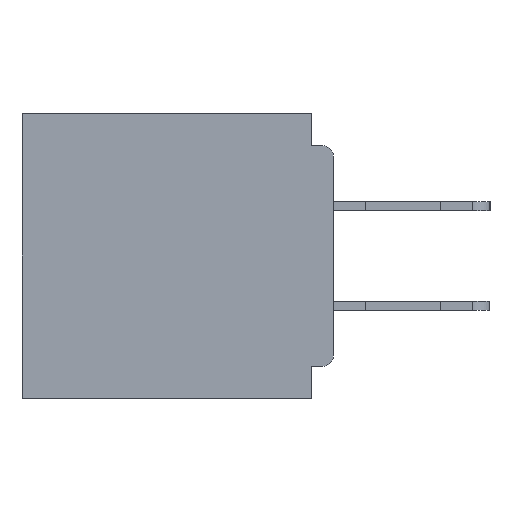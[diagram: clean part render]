
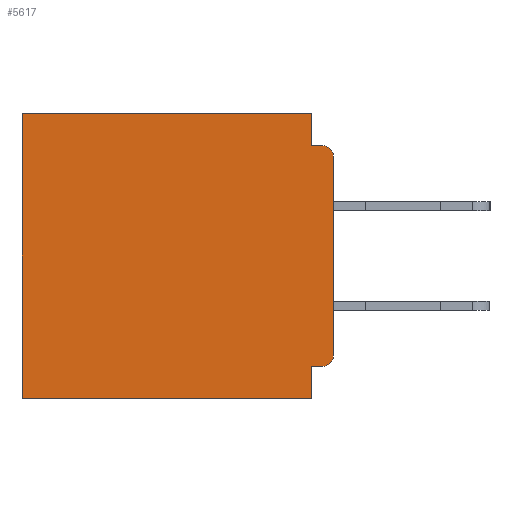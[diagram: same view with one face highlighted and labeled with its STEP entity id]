
A CAD part, left-side view. The second image highlights one B-rep face of the part: STEP entity #5617.
In plain terms, the highlighted planar face has unit normal (-1, 0, 0).
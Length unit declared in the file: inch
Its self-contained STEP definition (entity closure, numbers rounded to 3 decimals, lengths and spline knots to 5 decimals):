
#1037 = LINE ( 'NONE', #33477, #38557 ) ;
#1380 = DIRECTION ( 'NONE',  ( 0., -1., 0. ) ) ;
#1863 = EDGE_CURVE ( 'NONE', #27059, #33455, #26559, .T. ) ;
#2200 = DIRECTION ( 'NONE',  ( 1., 0., 0. ) ) ;
#4066 = EDGE_CURVE ( 'NONE', #7478, #38044, #1037, .T. ) ;
#4143 = CARTESIAN_POINT ( 'NONE',  ( 0.3, 0.015, -0.34 ) ) ;
#4720 = VERTEX_POINT ( 'NONE', #11070 ) ;
#5083 = FACE_OUTER_BOUND ( 'NONE', #17525, .T. ) ;
#5617 = ADVANCED_FACE ( 'NONE', ( #5083 ), #24714, .F. ) ;
#6187 = CARTESIAN_POINT ( 'NONE',  ( 0.3, 0., -0.4 ) ) ;
#6511 = CIRCLE ( 'NONE', #29868, 0.015 ) ;
#6643 = VERTEX_POINT ( 'NONE', #28253 ) ;
#7478 = VERTEX_POINT ( 'NONE', #33227 ) ;
#8003 = DIRECTION ( 'NONE',  ( 0., 0., -1. ) ) ;
#8514 = LINE ( 'NONE', #6187, #18417 ) ;
#8592 = EDGE_CURVE ( 'NONE', #28787, #31553, #8514, .T. ) ;
#9430 = CARTESIAN_POINT ( 'NONE',  ( 0.3, 0., -0.355 ) ) ;
#9519 = EDGE_CURVE ( 'NONE', #28787, #46571, #16006, .T. ) ;
#9896 = DIRECTION ( 'NONE',  ( 0., 1., 0. ) ) ;
#11070 = CARTESIAN_POINT ( 'NONE',  ( 0.3, 0.031, -0.355 ) ) ;
#11517 = ORIENTED_EDGE ( 'NONE', *, *, #4066, .F. ) ;
#15124 = CARTESIAN_POINT ( 'NONE',  ( 0.3, 0., -0.06 ) ) ;
#15495 = VECTOR ( 'NONE', #15635, 39.37008 ) ;
#15635 = DIRECTION ( 'NONE',  ( 0., 1., 0. ) ) ;
#16006 = CIRCLE ( 'NONE', #46215, 0.015 ) ;
#16523 = LINE ( 'NONE', #28769, #35234 ) ;
#17525 = EDGE_LOOP ( 'NONE', ( #47558, #17944, #19115, #11517, #26168, #48163, #24986, #31431, #34925, #23362 ) ) ;
#17944 = ORIENTED_EDGE ( 'NONE', *, *, #9519, .T. ) ;
#18105 = CARTESIAN_POINT ( 'NONE',  ( 0.3, 0.015, -0.06 ) ) ;
#18132 = LINE ( 'NONE', #9430, #26917 ) ;
#18162 = CARTESIAN_POINT ( 'NONE',  ( 0.3, 0., -0.34 ) ) ;
#18417 = VECTOR ( 'NONE', #32317, 39.37008 ) ;
#19115 = ORIENTED_EDGE ( 'NONE', *, *, #44430, .F. ) ;
#19328 = CARTESIAN_POINT ( 'NONE',  ( 0.3, 0.437, -0.4 ) ) ;
#19511 = EDGE_CURVE ( 'NONE', #30591, #4720, #18132, .T. ) ;
#20132 = VECTOR ( 'NONE', #9896, 39.37008 ) ;
#20237 = DIRECTION ( 'NONE',  ( 0., 0., -1. ) ) ;
#20951 = CARTESIAN_POINT ( 'NONE',  ( 0.3, 0., -0.4 ) ) ;
#21867 = DIRECTION ( 'NONE',  ( 0., 0., -1. ) ) ;
#22524 = CARTESIAN_POINT ( 'NONE',  ( 0.3, 0.031, -0.045 ) ) ;
#22567 = VECTOR ( 'NONE', #1380, 39.37008 ) ;
#23362 = ORIENTED_EDGE ( 'NONE', *, *, #47787, .T. ) ;
#23904 = CARTESIAN_POINT ( 'NONE',  ( 0.3, 0., -0.045 ) ) ;
#24247 = LINE ( 'NONE', #37978, #15495 ) ;
#24714 = PLANE ( 'NONE',  #38413 ) ;
#24986 = ORIENTED_EDGE ( 'NONE', *, *, #45618, .F. ) ;
#26168 = ORIENTED_EDGE ( 'NONE', *, *, #45929, .T. ) ;
#26559 = LINE ( 'NONE', #19328, #43955 ) ;
#26917 = VECTOR ( 'NONE', #39247, 39.37008 ) ;
#27059 = VERTEX_POINT ( 'NONE', #38459 ) ;
#28253 = CARTESIAN_POINT ( 'NONE',  ( 0.3, 0.031, -0.4 ) ) ;
#28473 = DIRECTION ( 'NONE',  ( 0., 0., -1. ) ) ;
#28769 = CARTESIAN_POINT ( 'NONE',  ( 0.3, 0.031, -0.4 ) ) ;
#28787 = VERTEX_POINT ( 'NONE', #15124 ) ;
#29868 = AXIS2_PLACEMENT_3D ( 'NONE', #4143, #30381, #8003 ) ;
#30093 = LINE ( 'NONE', #46945, #20132 ) ;
#30145 = EDGE_CURVE ( 'NONE', #4720, #6643, #16523, .T. ) ;
#30381 = DIRECTION ( 'NONE',  ( -1., 0., 0. ) ) ;
#30591 = VERTEX_POINT ( 'NONE', #38644 ) ;
#31431 = ORIENTED_EDGE ( 'NONE', *, *, #30145, .F. ) ;
#31553 = VERTEX_POINT ( 'NONE', #18162 ) ;
#32317 = DIRECTION ( 'NONE',  ( 0., 0., -1. ) ) ;
#32508 = DIRECTION ( 'NONE',  ( 0., 0., -1. ) ) ;
#33227 = CARTESIAN_POINT ( 'NONE',  ( 0.3, 0.031, 0. ) ) ;
#33455 = VERTEX_POINT ( 'NONE', #37112 ) ;
#33477 = CARTESIAN_POINT ( 'NONE',  ( 0.3, 0.031, 0. ) ) ;
#34925 = ORIENTED_EDGE ( 'NONE', *, *, #19511, .F. ) ;
#35234 = VECTOR ( 'NONE', #32508, 39.37008 ) ;
#37112 = CARTESIAN_POINT ( 'NONE',  ( 0.3, 0.437, -0.4 ) ) ;
#37245 = DIRECTION ( 'NONE',  ( 0., 0., -1. ) ) ;
#37978 = CARTESIAN_POINT ( 'NONE',  ( 0.3, 0., -0.4 ) ) ;
#38044 = VERTEX_POINT ( 'NONE', #22524 ) ;
#38413 = AXIS2_PLACEMENT_3D ( 'NONE', #20951, #2200, #28473 ) ;
#38459 = CARTESIAN_POINT ( 'NONE',  ( 0.3, 0.437, 0. ) ) ;
#38557 = VECTOR ( 'NONE', #37245, 39.37008 ) ;
#38644 = CARTESIAN_POINT ( 'NONE',  ( 0.3, 0.015, -0.355 ) ) ;
#39247 = DIRECTION ( 'NONE',  ( 0., 1., 0. ) ) ;
#41158 = LINE ( 'NONE', #23904, #22567 ) ;
#41942 = CARTESIAN_POINT ( 'NONE',  ( 0.3, 0.015, -0.045 ) ) ;
#43955 = VECTOR ( 'NONE', #20237, 39.37008 ) ;
#44124 = DIRECTION ( 'NONE',  ( -1., 0., 0. ) ) ;
#44430 = EDGE_CURVE ( 'NONE', #38044, #46571, #41158, .T. ) ;
#45618 = EDGE_CURVE ( 'NONE', #6643, #33455, #24247, .T. ) ;
#45929 = EDGE_CURVE ( 'NONE', #7478, #27059, #30093, .T. ) ;
#46215 = AXIS2_PLACEMENT_3D ( 'NONE', #18105, #44124, #21867 ) ;
#46571 = VERTEX_POINT ( 'NONE', #41942 ) ;
#46945 = CARTESIAN_POINT ( 'NONE',  ( 0.3, 0., 0. ) ) ;
#47558 = ORIENTED_EDGE ( 'NONE', *, *, #8592, .F. ) ;
#47787 = EDGE_CURVE ( 'NONE', #30591, #31553, #6511, .T. ) ;
#48163 = ORIENTED_EDGE ( 'NONE', *, *, #1863, .T. ) ;
